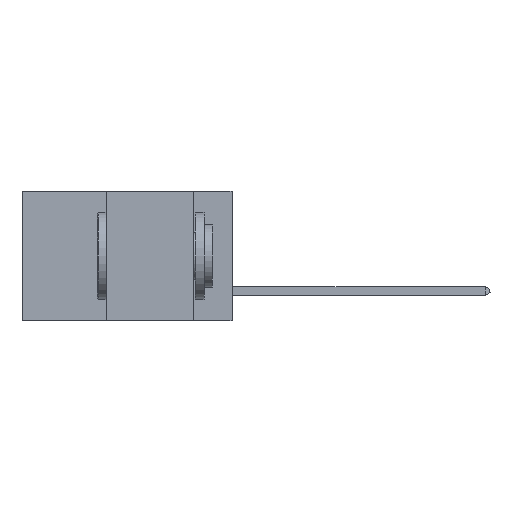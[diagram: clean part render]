
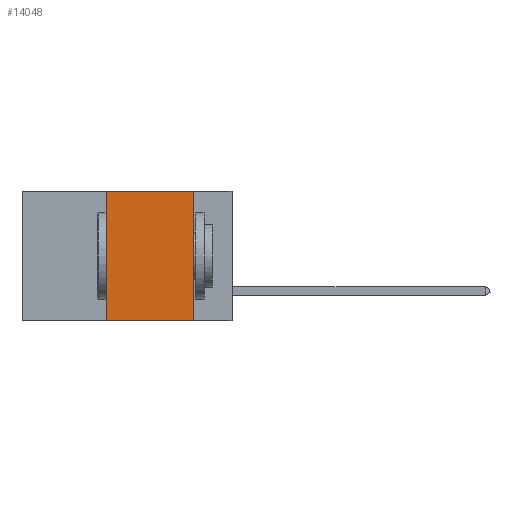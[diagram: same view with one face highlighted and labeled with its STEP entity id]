
A CAD part, left-side view. The second image highlights one B-rep face of the part: STEP entity #14048.
In plain terms, the highlighted planar face has unit normal (-1, 0, 0).
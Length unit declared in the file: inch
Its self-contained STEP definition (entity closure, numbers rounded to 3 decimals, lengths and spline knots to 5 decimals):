
#115 = CARTESIAN_POINT ( 'NONE',  ( 0., 0.11, -0.37 ) ) ;
#545 = DIRECTION ( 'NONE',  ( 0., 0., 1. ) ) ;
#1071 = VECTOR ( 'NONE', #4354, 39.37008 ) ;
#1098 = VERTEX_POINT ( 'NONE', #115 ) ;
#2401 = VERTEX_POINT ( 'NONE', #14261 ) ;
#2481 = LINE ( 'NONE', #7921, #1071 ) ;
#2614 = VECTOR ( 'NONE', #545, 39.37008 ) ;
#2981 = CARTESIAN_POINT ( 'NONE',  ( 0., 0.36, 0. ) ) ;
#3764 = AXIS2_PLACEMENT_3D ( 'NONE', #8142, #20481, #18786 ) ;
#4354 = DIRECTION ( 'NONE',  ( 0., 0., -1. ) ) ;
#4435 = EDGE_CURVE ( 'NONE', #13061, #21512, #21385, .T. ) ;
#4663 = EDGE_CURVE ( 'NONE', #13061, #1098, #7564, .T. ) ;
#5355 = DIRECTION ( 'NONE',  ( 0., -1., 0. ) ) ;
#7564 = LINE ( 'NONE', #10708, #17267 ) ;
#7921 = CARTESIAN_POINT ( 'NONE',  ( 0., 0.11, 0. ) ) ;
#8142 = CARTESIAN_POINT ( 'NONE',  ( 0., 0.6, 0. ) ) ;
#8239 = ORIENTED_EDGE ( 'NONE', *, *, #4663, .T. ) ;
#9023 = EDGE_CURVE ( 'NONE', #2401, #1098, #2481, .T. ) ;
#9323 = ORIENTED_EDGE ( 'NONE', *, *, #4435, .F. ) ;
#9920 = ORIENTED_EDGE ( 'NONE', *, *, #11509, .F. ) ;
#10708 = CARTESIAN_POINT ( 'NONE',  ( 0., 0.6, -0.37 ) ) ;
#11174 = CARTESIAN_POINT ( 'NONE',  ( 0., 0.36, 0. ) ) ;
#11509 = EDGE_CURVE ( 'NONE', #21512, #2401, #16458, .T. ) ;
#11804 = VECTOR ( 'NONE', #16396, 39.37008 ) ;
#12871 = CARTESIAN_POINT ( 'NONE',  ( 0., 0.6, 0. ) ) ;
#13061 = VERTEX_POINT ( 'NONE', #15229 ) ;
#14048 = ADVANCED_FACE ( 'NONE', ( #16568 ), #18703, .F. ) ;
#14261 = CARTESIAN_POINT ( 'NONE',  ( 0., 0.11, 0. ) ) ;
#15229 = CARTESIAN_POINT ( 'NONE',  ( 0., 0.36, -0.37 ) ) ;
#16396 = DIRECTION ( 'NONE',  ( 0., -1., 0. ) ) ;
#16458 = LINE ( 'NONE', #12871, #11804 ) ;
#16505 = EDGE_LOOP ( 'NONE', ( #21634, #9920, #9323, #8239 ) ) ;
#16568 = FACE_OUTER_BOUND ( 'NONE', #16505, .T. ) ;
#17267 = VECTOR ( 'NONE', #5355, 39.37008 ) ;
#18703 = PLANE ( 'NONE',  #3764 ) ;
#18786 = DIRECTION ( 'NONE',  ( 0., 0., -1. ) ) ;
#20481 = DIRECTION ( 'NONE',  ( 1., 0., 0. ) ) ;
#21385 = LINE ( 'NONE', #11174, #2614 ) ;
#21512 = VERTEX_POINT ( 'NONE', #2981 ) ;
#21634 = ORIENTED_EDGE ( 'NONE', *, *, #9023, .F. ) ;
